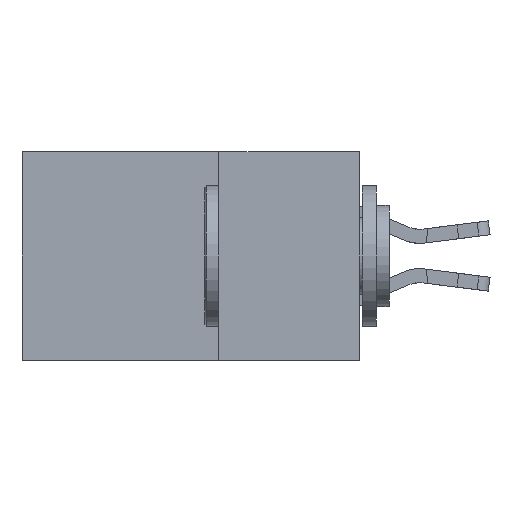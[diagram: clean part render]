
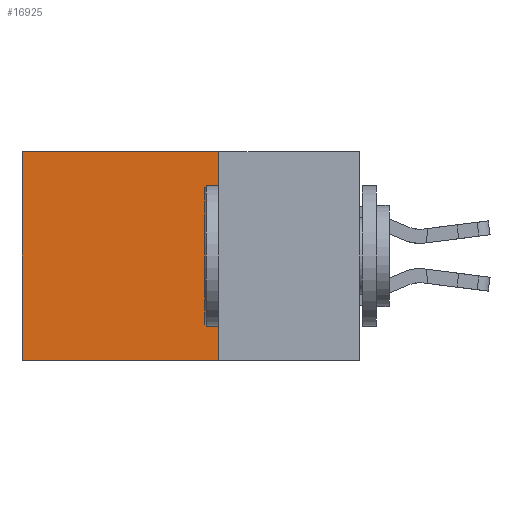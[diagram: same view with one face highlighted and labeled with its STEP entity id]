
A CAD part, left-side view. The second image highlights one B-rep face of the part: STEP entity #16925.
In plain terms, the highlighted planar face has unit normal (-1, 0, 0).
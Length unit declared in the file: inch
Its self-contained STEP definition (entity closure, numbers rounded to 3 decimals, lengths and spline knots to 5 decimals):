
#1664 = CARTESIAN_POINT ( 'NONE',  ( 0.2875, 0.25, 0. ) ) ;
#2244 = EDGE_LOOP ( 'NONE', ( #11281, #7002, #10042, #5154 ) ) ;
#4607 = DIRECTION ( 'NONE',  ( 0., 0., -1. ) ) ;
#4781 = EDGE_CURVE ( 'NONE', #15300, #4874, #30116, .T. ) ;
#4874 = VERTEX_POINT ( 'NONE', #16382 ) ;
#5154 = ORIENTED_EDGE ( 'NONE', *, *, #5687, .T. ) ;
#5542 = DIRECTION ( 'NONE',  ( 0., 1., 0. ) ) ;
#5687 = EDGE_CURVE ( 'NONE', #32981, #15300, #17502, .T. ) ;
#7002 = ORIENTED_EDGE ( 'NONE', *, *, #33038, .F. ) ;
#9994 = CARTESIAN_POINT ( 'NONE',  ( 0.2875, 0.25, -0.37 ) ) ;
#10042 = ORIENTED_EDGE ( 'NONE', *, *, #32407, .F. ) ;
#10241 = PLANE ( 'NONE',  #15726 ) ;
#11281 = ORIENTED_EDGE ( 'NONE', *, *, #4781, .T. ) ;
#13135 = DIRECTION ( 'NONE',  ( 1., 0., 0. ) ) ;
#15300 = VERTEX_POINT ( 'NONE', #36126 ) ;
#15330 = VECTOR ( 'NONE', #32796, 39.37008 ) ;
#15726 = AXIS2_PLACEMENT_3D ( 'NONE', #18713, #13135, #32665 ) ;
#16382 = CARTESIAN_POINT ( 'NONE',  ( 0.2875, 0.6, -0.37 ) ) ;
#16871 = VERTEX_POINT ( 'NONE', #9994 ) ;
#16925 = ADVANCED_FACE ( 'NONE', ( #31844 ), #10241, .F. ) ;
#17502 = LINE ( 'NONE', #33571, #24051 ) ;
#18558 = CARTESIAN_POINT ( 'NONE',  ( 0.2875, 0.25, -0.37 ) ) ;
#18713 = CARTESIAN_POINT ( 'NONE',  ( 0.2875, 0.25, 0. ) ) ;
#19955 = LINE ( 'NONE', #1664, #33822 ) ;
#23836 = LINE ( 'NONE', #18558, #30304 ) ;
#24051 = VECTOR ( 'NONE', #5542, 39.37008 ) ;
#24284 = DIRECTION ( 'NONE',  ( 0., 1., 0. ) ) ;
#29985 = CARTESIAN_POINT ( 'NONE',  ( 0.2875, 0.6, 0. ) ) ;
#30116 = LINE ( 'NONE', #29985, #15330 ) ;
#30304 = VECTOR ( 'NONE', #24284, 39.37008 ) ;
#31844 = FACE_OUTER_BOUND ( 'NONE', #2244, .T. ) ;
#32407 = EDGE_CURVE ( 'NONE', #32981, #16871, #19955, .T. ) ;
#32665 = DIRECTION ( 'NONE',  ( 0., 0., -1. ) ) ;
#32796 = DIRECTION ( 'NONE',  ( 0., 0., -1. ) ) ;
#32981 = VERTEX_POINT ( 'NONE', #35035 ) ;
#33038 = EDGE_CURVE ( 'NONE', #16871, #4874, #23836, .T. ) ;
#33571 = CARTESIAN_POINT ( 'NONE',  ( 0.2875, 0.25, 0. ) ) ;
#33822 = VECTOR ( 'NONE', #4607, 39.37008 ) ;
#35035 = CARTESIAN_POINT ( 'NONE',  ( 0.2875, 0.25, 0. ) ) ;
#36126 = CARTESIAN_POINT ( 'NONE',  ( 0.2875, 0.6, 0. ) ) ;
